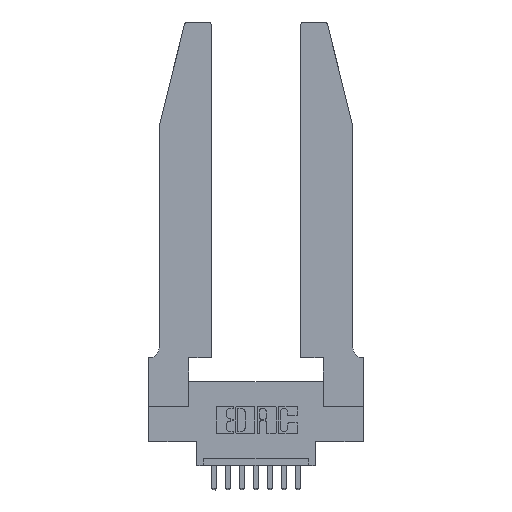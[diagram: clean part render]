
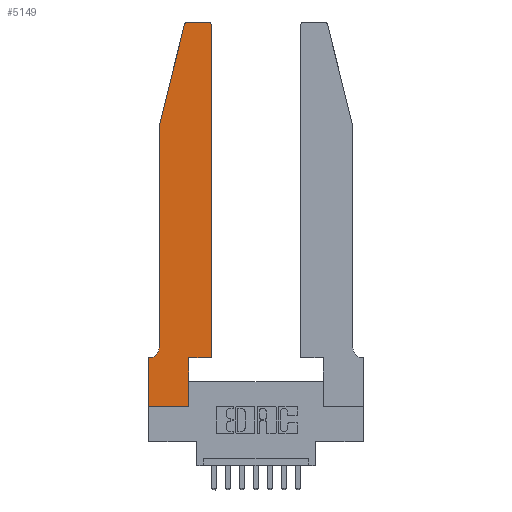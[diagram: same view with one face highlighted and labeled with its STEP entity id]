
A CAD part, top view. The second image highlights one B-rep face of the part: STEP entity #5149.
In plain terms, the highlighted planar face has unit normal (0, 0, 1).
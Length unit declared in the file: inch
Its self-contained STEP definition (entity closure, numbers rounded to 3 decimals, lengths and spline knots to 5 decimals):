
#4 = CIRCLE ( 'NONE', #2450, 0.03 ) ;
#73 = CARTESIAN_POINT ( 'NONE',  ( 0., 0., 0.37 ) ) ;
#152 = EDGE_CURVE ( 'NONE', #13778, #10242, #11453, .T. ) ;
#245 = LINE ( 'NONE', #73, #4446 ) ;
#319 = CARTESIAN_POINT ( 'NONE',  ( 0., 0., 0.37 ) ) ;
#447 = DIRECTION ( 'NONE',  ( 0., 0., 1. ) ) ;
#458 = PLANE ( 'NONE',  #2934 ) ;
#710 = VECTOR ( 'NONE', #4095, 39.37008 ) ;
#944 = VERTEX_POINT ( 'NONE', #12508 ) ;
#1067 = VECTOR ( 'NONE', #11462, 39.37008 ) ;
#1079 = EDGE_CURVE ( 'NONE', #10242, #9802, #5328, .T. ) ;
#1117 = CARTESIAN_POINT ( 'NONE',  ( 0.2605, 2.75, 0.37 ) ) ;
#1165 = CARTESIAN_POINT ( 'NONE',  ( 0.2865, 0.35, 0.37 ) ) ;
#1573 = EDGE_CURVE ( 'NONE', #9802, #5104, #12149, .T. ) ;
#1741 = CARTESIAN_POINT ( 'NONE',  ( 0.0755, 2., 0.37 ) ) ;
#1748 = ORIENTED_EDGE ( 'NONE', *, *, #9878, .T. ) ;
#2123 = CARTESIAN_POINT ( 'NONE',  ( 0.25487, 2.72718, 0.37 ) ) ;
#2450 = AXIS2_PLACEMENT_3D ( 'NONE', #8459, #10898, #2849 ) ;
#2562 = CARTESIAN_POINT ( 'NONE',  ( 0.4205, 2.75, 0.37 ) ) ;
#2573 = ORIENTED_EDGE ( 'NONE', *, *, #12548, .T. ) ;
#2706 = VERTEX_POINT ( 'NONE', #2123 ) ;
#2849 = DIRECTION ( 'NONE',  ( 1., 0., 0. ) ) ;
#2902 = CARTESIAN_POINT ( 'NONE',  ( 0.0755, 2., 0.37 ) ) ;
#2919 = VERTEX_POINT ( 'NONE', #2562 ) ;
#2934 = AXIS2_PLACEMENT_3D ( 'NONE', #9778, #12136, #5182 ) ;
#3158 = LINE ( 'NONE', #1741, #14880 ) ;
#3277 = VERTEX_POINT ( 'NONE', #13910 ) ;
#3293 = DIRECTION ( 'NONE',  ( -1., 0., 0. ) ) ;
#3413 = EDGE_CURVE ( 'NONE', #7153, #2706, #4, .T. ) ;
#3653 = DIRECTION ( 'NONE',  ( 0., -1., 0. ) ) ;
#4095 = DIRECTION ( 'NONE',  ( -1., 0., 0. ) ) ;
#4104 = VECTOR ( 'NONE', #9584, 39.37008 ) ;
#4119 = DIRECTION ( 'NONE',  ( -0.239, -0.971, 0. ) ) ;
#4339 = VECTOR ( 'NONE', #4119, 39.37008 ) ;
#4446 = VECTOR ( 'NONE', #3653, 39.37008 ) ;
#4518 = VERTEX_POINT ( 'NONE', #6819 ) ;
#4842 = CARTESIAN_POINT ( 'NONE',  ( 0.2865, 0.35, 0.37 ) ) ;
#4936 = ORIENTED_EDGE ( 'NONE', *, *, #7461, .T. ) ;
#5057 = LINE ( 'NONE', #2902, #4339 ) ;
#5104 = VERTEX_POINT ( 'NONE', #7797 ) ;
#5149 = ADVANCED_FACE ( 'NONE', ( #8108 ), #458, .T. ) ;
#5182 = DIRECTION ( 'NONE',  ( 1., 0., 0. ) ) ;
#5295 = EDGE_CURVE ( 'NONE', #4518, #944, #11722, .T. ) ;
#5328 = LINE ( 'NONE', #14015, #9605 ) ;
#5588 = LINE ( 'NONE', #1117, #1067 ) ;
#5781 = EDGE_CURVE ( 'NONE', #944, #9021, #10624, .T. ) ;
#6332 = EDGE_LOOP ( 'NONE', ( #1748, #12051, #13068, #8796, #9611, #14080, #2573, #4936, #14806, #8297, #7860, #8745 ) ) ;
#6819 = CARTESIAN_POINT ( 'NONE',  ( 0.0755, 0.42, 0.37 ) ) ;
#7090 = CIRCLE ( 'NONE', #9944, 0.03 ) ;
#7153 = VERTEX_POINT ( 'NONE', #14374 ) ;
#7461 = EDGE_CURVE ( 'NONE', #3277, #13778, #13851, .T. ) ;
#7797 = CARTESIAN_POINT ( 'NONE',  ( 0.4505, 2.72, 0.37 ) ) ;
#7800 = DIRECTION ( 'NONE',  ( 0., 0., -1. ) ) ;
#7860 = ORIENTED_EDGE ( 'NONE', *, *, #1573, .T. ) ;
#8108 = FACE_OUTER_BOUND ( 'NONE', #6332, .T. ) ;
#8297 = ORIENTED_EDGE ( 'NONE', *, *, #1079, .T. ) ;
#8459 = CARTESIAN_POINT ( 'NONE',  ( 0.284, 2.72, 0.37 ) ) ;
#8467 = CARTESIAN_POINT ( 'NONE',  ( 0.4505, 0.35, 0.37 ) ) ;
#8512 = CARTESIAN_POINT ( 'NONE',  ( 0.4205, 2.72, 0.37 ) ) ;
#8592 = CARTESIAN_POINT ( 'NONE',  ( 0.0755, 0.35, 0.37 ) ) ;
#8745 = ORIENTED_EDGE ( 'NONE', *, *, #9425, .T. ) ;
#8796 = ORIENTED_EDGE ( 'NONE', *, *, #9407, .T. ) ;
#9021 = VERTEX_POINT ( 'NONE', #14061 ) ;
#9407 = EDGE_CURVE ( 'NONE', #10236, #4518, #3158, .T. ) ;
#9425 = EDGE_CURVE ( 'NONE', #5104, #2919, #7090, .T. ) ;
#9545 = AXIS2_PLACEMENT_3D ( 'NONE', #13581, #7800, #3293 ) ;
#9584 = DIRECTION ( 'NONE',  ( 1., 0., 0. ) ) ;
#9605 = VECTOR ( 'NONE', #11587, 39.37008 ) ;
#9611 = ORIENTED_EDGE ( 'NONE', *, *, #5295, .T. ) ;
#9710 = CARTESIAN_POINT ( 'NONE',  ( 0.2865, 0., 0.37 ) ) ;
#9778 = CARTESIAN_POINT ( 'NONE',  ( 0., 0.35, 0.37 ) ) ;
#9779 = EDGE_CURVE ( 'NONE', #2706, #10236, #5057, .T. ) ;
#9802 = VERTEX_POINT ( 'NONE', #8467 ) ;
#9878 = EDGE_CURVE ( 'NONE', #2919, #7153, #5588, .T. ) ;
#9944 = AXIS2_PLACEMENT_3D ( 'NONE', #8512, #447, #10752 ) ;
#10236 = VERTEX_POINT ( 'NONE', #11155 ) ;
#10242 = VERTEX_POINT ( 'NONE', #1165 ) ;
#10624 = LINE ( 'NONE', #8592, #710 ) ;
#10752 = DIRECTION ( 'NONE',  ( 1., 0., 0. ) ) ;
#10764 = DIRECTION ( 'NONE',  ( 0., 1., 0. ) ) ;
#10898 = DIRECTION ( 'NONE',  ( 0., 0., 1. ) ) ;
#10964 = DIRECTION ( 'NONE',  ( 0., -1., 0. ) ) ;
#11155 = CARTESIAN_POINT ( 'NONE',  ( 0.0755, 2., 0.37 ) ) ;
#11453 = LINE ( 'NONE', #4842, #12724 ) ;
#11462 = DIRECTION ( 'NONE',  ( -1., 0., 0. ) ) ;
#11587 = DIRECTION ( 'NONE',  ( 1., 0., 0. ) ) ;
#11722 = CIRCLE ( 'NONE', #9545, 0.07 ) ;
#12051 = ORIENTED_EDGE ( 'NONE', *, *, #3413, .T. ) ;
#12136 = DIRECTION ( 'NONE',  ( 0., 0., 1. ) ) ;
#12149 = LINE ( 'NONE', #14653, #12881 ) ;
#12508 = CARTESIAN_POINT ( 'NONE',  ( 0.0055, 0.35, 0.37 ) ) ;
#12548 = EDGE_CURVE ( 'NONE', #9021, #3277, #245, .T. ) ;
#12724 = VECTOR ( 'NONE', #10764, 39.37008 ) ;
#12881 = VECTOR ( 'NONE', #14705, 39.37008 ) ;
#13068 = ORIENTED_EDGE ( 'NONE', *, *, #9779, .T. ) ;
#13581 = CARTESIAN_POINT ( 'NONE',  ( 0.0055, 0.42, 0.37 ) ) ;
#13778 = VERTEX_POINT ( 'NONE', #9710 ) ;
#13851 = LINE ( 'NONE', #319, #4104 ) ;
#13910 = CARTESIAN_POINT ( 'NONE',  ( 0., 0., 0.37 ) ) ;
#14015 = CARTESIAN_POINT ( 'NONE',  ( 0.4505, 0.35, 0.37 ) ) ;
#14061 = CARTESIAN_POINT ( 'NONE',  ( 0., 0.35, 0.37 ) ) ;
#14080 = ORIENTED_EDGE ( 'NONE', *, *, #5781, .T. ) ;
#14374 = CARTESIAN_POINT ( 'NONE',  ( 0.284, 2.75, 0.37 ) ) ;
#14653 = CARTESIAN_POINT ( 'NONE',  ( 0.4505, 0.35, 0.37 ) ) ;
#14705 = DIRECTION ( 'NONE',  ( 0., 1., 0. ) ) ;
#14806 = ORIENTED_EDGE ( 'NONE', *, *, #152, .T. ) ;
#14880 = VECTOR ( 'NONE', #10964, 39.37008 ) ;
